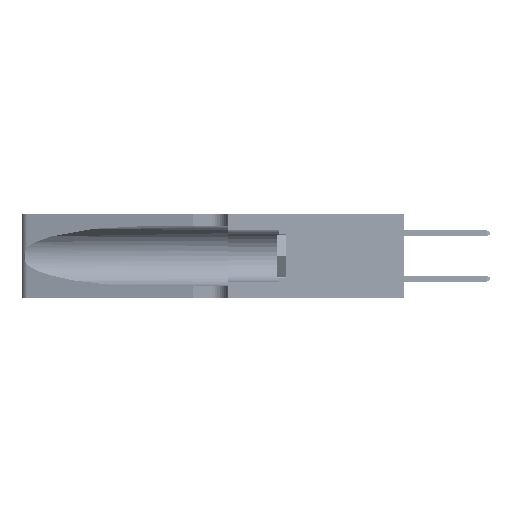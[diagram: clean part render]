
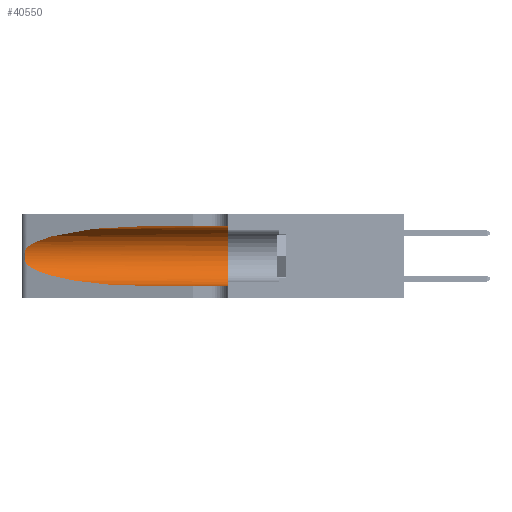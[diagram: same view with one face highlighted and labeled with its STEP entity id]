
A CAD part, left-side view. The second image highlights one B-rep face of the part: STEP entity #40550.
In plain terms, the highlighted cylindrical face has radius 3.308 mm (diameter 6.617 mm), a partial arc.
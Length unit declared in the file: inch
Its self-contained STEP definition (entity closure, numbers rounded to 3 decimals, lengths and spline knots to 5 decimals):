
#104 =( BOUNDED_CURVE ( )  B_SPLINE_CURVE ( 3, ( #39430, #43149, #23347, #6661 ),
 .UNSPECIFIED., .F., .F. ) 
 B_SPLINE_CURVE_WITH_KNOTS ( ( 4, 4 ),
 ( 1.5708, 2.84003 ),
 .UNSPECIFIED. ) 
 CURVE ( )  GEOMETRIC_REPRESENTATION_ITEM ( )  RATIONAL_B_SPLINE_CURVE ( ( 1., 0.87, 0.87, 1. ) ) 
 REPRESENTATION_ITEM ( '' )  );
#339 = CARTESIAN_POINT ( 'NONE',  ( 0.25639, 1.23186, 0.15144 ) ) ;
#1876 = EDGE_CURVE ( 'NONE', #20082, #26910, #12813, .T. ) ;
#3149 = CARTESIAN_POINT ( 'NONE',  ( 0.2373, 1.15595, 0.08982 ) ) ;
#4634 = DIRECTION ( 'NONE',  ( 0., 0., 1. ) ) ;
#5565 = CARTESIAN_POINT ( 'NONE',  ( 0.26018, 1.23835, 0.19895 ) ) ;
#5938 = FACE_OUTER_BOUND ( 'NONE', #18117, .T. ) ;
#6131 = ORIENTED_EDGE ( 'NONE', *, *, #43534, .T. ) ;
#6319 = CARTESIAN_POINT ( 'NONE',  ( 0.1305, 0.35, 0.05475 ) ) ;
#6661 = CARTESIAN_POINT ( 'NONE',  ( 0.25487, 1.22718, 0.22369 ) ) ;
#6833 = CARTESIAN_POINT ( 'NONE',  ( 0.25487, 1.22718, 0.14631 ) ) ;
#9953 = DIRECTION ( 'NONE',  ( 0., -1., 0. ) ) ;
#10820 = EDGE_CURVE ( 'NONE', #14278, #14883, #104, .T. ) ;
#11281 = CARTESIAN_POINT ( 'NONE',  ( 0.25487, 1.22718, 0.22369 ) ) ;
#11364 = VECTOR ( 'NONE', #42260, 39.37008 ) ;
#11561 = CARTESIAN_POINT ( 'NONE',  ( 0.25487, 1.22718, 0.22369 ) ) ;
#12351 = AXIS2_PLACEMENT_3D ( 'NONE', #48509, #32644, #4634 ) ;
#12482 = CARTESIAN_POINT ( 'NONE',  ( 0.25555, 1.22993, 0.14849 ) ) ;
#12813 = CIRCLE ( 'NONE', #12351, 0.13025 ) ;
#14278 = VERTEX_POINT ( 'NONE', #20592 ) ;
#14352 = CARTESIAN_POINT ( 'NONE',  ( 0.1305, 0.72297, 0.05475 ) ) ;
#14518 = ORIENTED_EDGE ( 'NONE', *, *, #1876, .F. ) ;
#14883 = VERTEX_POINT ( 'NONE', #11561 ) ;
#14924 = CARTESIAN_POINT ( 'NONE',  ( 0.18966, 0.96281, 0.05475 ) ) ;
#16388 = VERTEX_POINT ( 'NONE', #14352 ) ;
#16470 = EDGE_CURVE ( 'NONE', #14883, #36850, #29821, .T. ) ;
#16569 = CARTESIAN_POINT ( 'NONE',  ( 0.1305, 1.61858, 0.185 ) ) ;
#17725 = VECTOR ( 'NONE', #9953, 39.37008 ) ;
#18117 = EDGE_LOOP ( 'NONE', ( #27191, #27677, #6131, #24423, #14518, #48764 ) ) ;
#18234 = EDGE_CURVE ( 'NONE', #16388, #26910, #39161, .T. ) ;
#18983 = LINE ( 'NONE', #45935, #17725 ) ;
#20082 = VERTEX_POINT ( 'NONE', #23650 ) ;
#20528 = CARTESIAN_POINT ( 'NONE',  ( 0.25854, 1.2359, 0.20912 ) ) ;
#20592 = CARTESIAN_POINT ( 'NONE',  ( 0.1305, 0.72297, 0.31525 ) ) ;
#22095 = CARTESIAN_POINT ( 'NONE',  ( 0.25789, 1.23486, 0.15765 ) ) ;
#23347 = CARTESIAN_POINT ( 'NONE',  ( 0.2373, 1.15595, 0.28018 ) ) ;
#23650 = CARTESIAN_POINT ( 'NONE',  ( 0.1305, 0.35, 0.31525 ) ) ;
#23756 = CARTESIAN_POINT ( 'NONE',  ( 0.25787, 1.23484, 0.2124 ) ) ;
#24423 = ORIENTED_EDGE ( 'NONE', *, *, #18234, .T. ) ;
#26910 = VERTEX_POINT ( 'NONE', #6319 ) ;
#27080 = CARTESIAN_POINT ( 'NONE',  ( 0.1305, 0.72297, 0.05475 ) ) ;
#27191 = ORIENTED_EDGE ( 'NONE', *, *, #10820, .T. ) ;
#27677 = ORIENTED_EDGE ( 'NONE', *, *, #16470, .T. ) ;
#29821 = B_SPLINE_CURVE_WITH_KNOTS ( 'NONE', 3,
 ( #11281, #49862, #31141, #23756, #20528, #5565, #32856, #37615, #30163, #50447, #22095, #339, #12482, #6833 ),
 .UNSPECIFIED., .F., .F.,
 ( 4, 2, 2, 2, 2, 2, 4 ),
 ( 0., 0.00027, 0.00053, 0.00107, 0.0016, 0.00187, 0.00214 ),
 .UNSPECIFIED. ) ;
#30163 = CARTESIAN_POINT ( 'NONE',  ( 0.26017, 1.23833, 0.17102 ) ) ;
#30650 = CARTESIAN_POINT ( 'NONE',  ( 0.25487, 1.22718, 0.14631 ) ) ;
#31141 = CARTESIAN_POINT ( 'NONE',  ( 0.25639, 1.23184, 0.21858 ) ) ;
#32644 = DIRECTION ( 'NONE',  ( 0., 1., 0. ) ) ;
#32856 = CARTESIAN_POINT ( 'NONE',  ( 0.26075, 1.23896, 0.19203 ) ) ;
#34401 =( BOUNDED_CURVE ( )  B_SPLINE_CURVE ( 3, ( #46673, #3149, #14924, #27080 ),
 .UNSPECIFIED., .F., .T. ) 
 B_SPLINE_CURVE_WITH_KNOTS ( ( 4, 4 ),
 ( 3.44316, 4.71239 ),
 .UNSPECIFIED. ) 
 CURVE ( )  GEOMETRIC_REPRESENTATION_ITEM ( )  RATIONAL_B_SPLINE_CURVE ( ( 1., 0.87, 0.87, 1. ) ) 
 REPRESENTATION_ITEM ( '' )  );
#36850 = VERTEX_POINT ( 'NONE', #30650 ) ;
#37212 = DIRECTION ( 'NONE',  ( 0., -1., 0. ) ) ;
#37615 = CARTESIAN_POINT ( 'NONE',  ( 0.26075, 1.23896, 0.178 ) ) ;
#37805 = EDGE_CURVE ( 'NONE', #14278, #20082, #18983, .T. ) ;
#39161 = LINE ( 'NONE', #50538, #11364 ) ;
#39430 = CARTESIAN_POINT ( 'NONE',  ( 0.1305, 0.72297, 0.31525 ) ) ;
#40550 = ADVANCED_FACE ( 'NONE', ( #5938 ), #46288, .F. ) ;
#42260 = DIRECTION ( 'NONE',  ( 0., -1., 0. ) ) ;
#42754 = AXIS2_PLACEMENT_3D ( 'NONE', #16569, #37212, #44758 ) ;
#43149 = CARTESIAN_POINT ( 'NONE',  ( 0.18966, 0.96281, 0.31525 ) ) ;
#43534 = EDGE_CURVE ( 'NONE', #36850, #16388, #34401, .T. ) ;
#44758 = DIRECTION ( 'NONE',  ( 0., 0., -1. ) ) ;
#45935 = CARTESIAN_POINT ( 'NONE',  ( 0.1305, 1.61858, 0.31525 ) ) ;
#46288 = CYLINDRICAL_SURFACE ( 'NONE', #42754, 0.13025 ) ;
#46673 = CARTESIAN_POINT ( 'NONE',  ( 0.25487, 1.22718, 0.14631 ) ) ;
#48509 = CARTESIAN_POINT ( 'NONE',  ( 0.1305, 0.35, 0.185 ) ) ;
#48764 = ORIENTED_EDGE ( 'NONE', *, *, #37805, .F. ) ;
#49862 = CARTESIAN_POINT ( 'NONE',  ( 0.25555, 1.22994, 0.2215 ) ) ;
#50447 = CARTESIAN_POINT ( 'NONE',  ( 0.25856, 1.23593, 0.16098 ) ) ;
#50538 = CARTESIAN_POINT ( 'NONE',  ( 0.1305, 1.61858, 0.05475 ) ) ;
